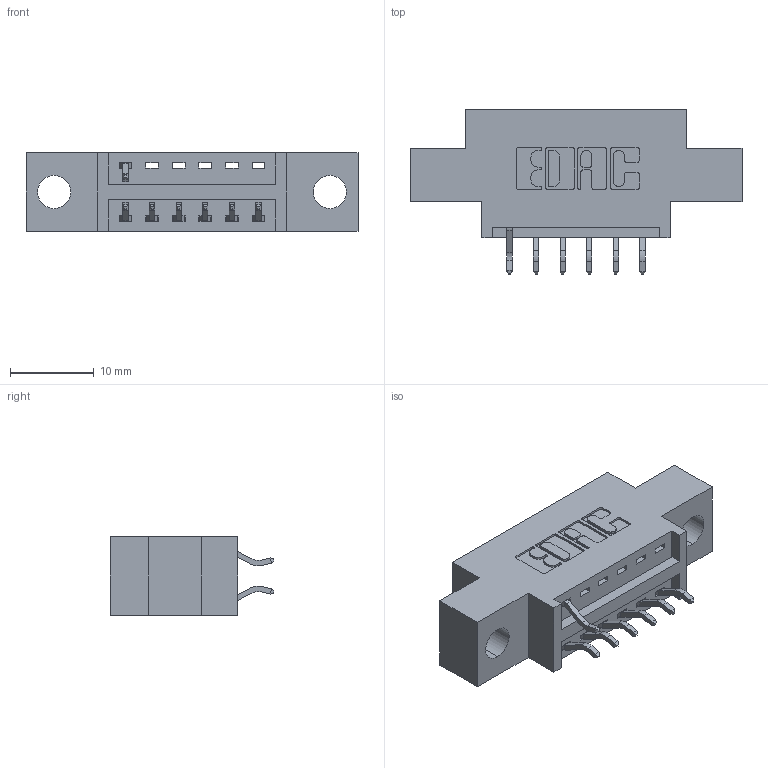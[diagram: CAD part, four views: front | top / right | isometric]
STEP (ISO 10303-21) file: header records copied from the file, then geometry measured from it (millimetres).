
FILE_DESCRIPTION (( 'STEP AP203' ), '1' );
FILE_NAME ('346-012-556-804.STEP', '2018-08-19T22:54:49', ( '' ), ( '' ), 'SwSTEP 2.0', 'SolidWorks 2016', '' );
FILE_SCHEMA (( 'CONFIG_CONTROL_DESIGN' ));
Length unit declared in the file: inch
Products named in the file (3): 346 Part_0.170 Offset - 0.156 Dia-TH; 345-292-001_556 Tail; 346-012-556-804
Assembly tree (8 placements, depth 2):
  346-012-556-804
    346 Part_0.170 Offset - 0.156 Dia-TH
    345-292-001_556 Tail  x7
Bounding box: 39.62 x 19.57 x 9.4 mm (x, y, z)
Volume: 3296.5 mm3; surface area: 3692.4 mm2
Topology: 8 solids, 8 shells, 562 faces, 1657 edges, 1094 vertices
Faces by surface type: plane 378, cylinder 184
Entity records: 8957 total; most frequent: CARTESIAN_POINT 1563, ORIENTED_EDGE 1490, DIRECTION 1411, EDGE_CURVE 745, VECTOR 581, LINE 581, VERTEX_POINT 494, AXIS2_PLACEMENT_3D 415
